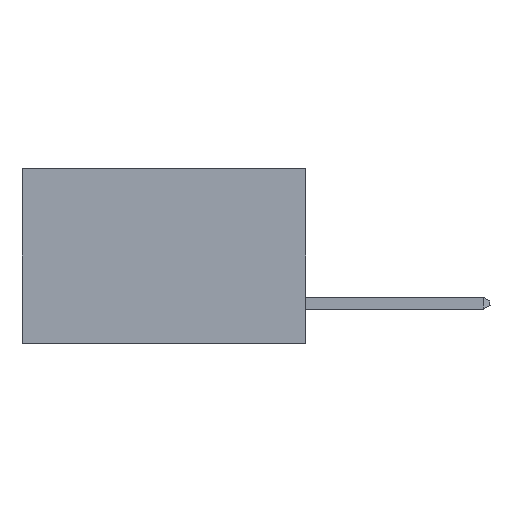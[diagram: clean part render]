
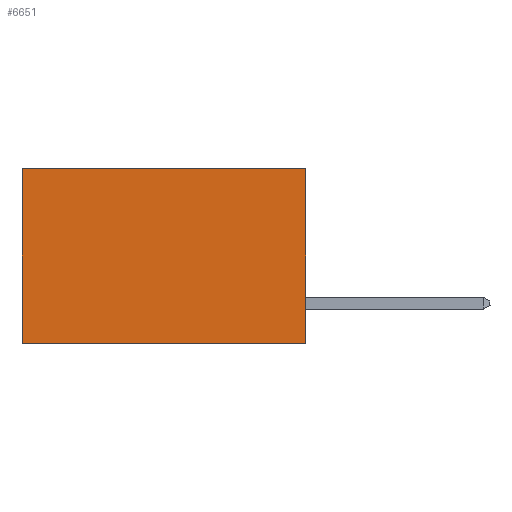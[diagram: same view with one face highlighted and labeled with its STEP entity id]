
A CAD part, left-side view. The second image highlights one B-rep face of the part: STEP entity #6651.
In plain terms, the highlighted planar face has unit normal (-1, 0, 0).
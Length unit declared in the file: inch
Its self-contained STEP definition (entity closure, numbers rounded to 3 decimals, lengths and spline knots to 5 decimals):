
#157 = LINE ( 'NONE', #1084, #6384 ) ;
#491 = AXIS2_PLACEMENT_3D ( 'NONE', #9232, #3219, #8125 ) ;
#1038 = ORIENTED_EDGE ( 'NONE', *, *, #1362, .T. ) ;
#1084 = CARTESIAN_POINT ( 'NONE',  ( 0.298, 0., 0. ) ) ;
#1193 = EDGE_CURVE ( 'NONE', #4935, #9348, #157, .T. ) ;
#1199 = DIRECTION ( 'NONE',  ( 0., 0., -1. ) ) ;
#1362 = EDGE_CURVE ( 'NONE', #9348, #6252, #2111, .T. ) ;
#1525 = VECTOR ( 'NONE', #2015, 39.37008 ) ;
#2015 = DIRECTION ( 'NONE',  ( 0., 1., 0. ) ) ;
#2111 = LINE ( 'NONE', #8564, #6043 ) ;
#2740 = EDGE_CURVE ( 'NONE', #3377, #6252, #8763, .T. ) ;
#2768 = EDGE_CURVE ( 'NONE', #4935, #3377, #4928, .T. ) ;
#2975 = ORIENTED_EDGE ( 'NONE', *, *, #2740, .F. ) ;
#3041 = ORIENTED_EDGE ( 'NONE', *, *, #2768, .F. ) ;
#3090 = ORIENTED_EDGE ( 'NONE', *, *, #1193, .T. ) ;
#3103 = CARTESIAN_POINT ( 'NONE',  ( 0.298, 0., 0. ) ) ;
#3219 = DIRECTION ( 'NONE',  ( 1., 0., 0. ) ) ;
#3231 = CARTESIAN_POINT ( 'NONE',  ( 0.298, 0.6, 0. ) ) ;
#3377 = VERTEX_POINT ( 'NONE', #4875 ) ;
#3726 = DIRECTION ( 'NONE',  ( 0., 1., 0. ) ) ;
#4447 = CARTESIAN_POINT ( 'NONE',  ( 0.298, 0.6, -0.37 ) ) ;
#4484 = FACE_OUTER_BOUND ( 'NONE', #7426, .T. ) ;
#4875 = CARTESIAN_POINT ( 'NONE',  ( 0.298, 0., -0.37 ) ) ;
#4928 = LINE ( 'NONE', #6566, #8217 ) ;
#4935 = VERTEX_POINT ( 'NONE', #3103 ) ;
#5926 = DIRECTION ( 'NONE',  ( 0., 0., -1. ) ) ;
#6043 = VECTOR ( 'NONE', #5926, 39.37008 ) ;
#6252 = VERTEX_POINT ( 'NONE', #4447 ) ;
#6384 = VECTOR ( 'NONE', #3726, 39.37008 ) ;
#6566 = CARTESIAN_POINT ( 'NONE',  ( 0.298, 0., 0. ) ) ;
#6651 = ADVANCED_FACE ( 'NONE', ( #4484 ), #9262, .F. ) ;
#7426 = EDGE_LOOP ( 'NONE', ( #1038, #2975, #3041, #3090 ) ) ;
#8125 = DIRECTION ( 'NONE',  ( 0., 0., -1. ) ) ;
#8217 = VECTOR ( 'NONE', #1199, 39.37008 ) ;
#8377 = CARTESIAN_POINT ( 'NONE',  ( 0.298, 0., -0.37 ) ) ;
#8564 = CARTESIAN_POINT ( 'NONE',  ( 0.298, 0.6, 0. ) ) ;
#8763 = LINE ( 'NONE', #8377, #1525 ) ;
#9232 = CARTESIAN_POINT ( 'NONE',  ( 0.298, 0., 0. ) ) ;
#9262 = PLANE ( 'NONE',  #491 ) ;
#9348 = VERTEX_POINT ( 'NONE', #3231 ) ;
